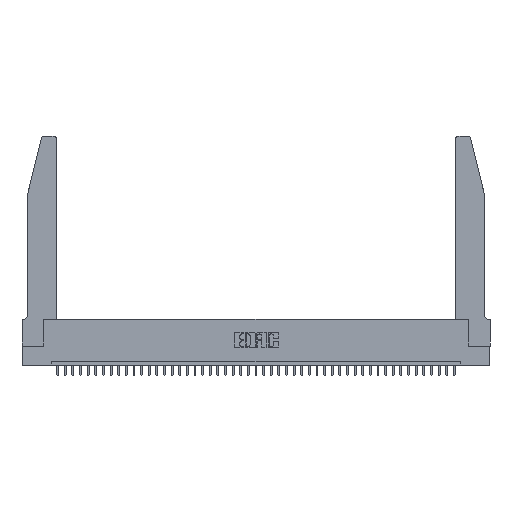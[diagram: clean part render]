
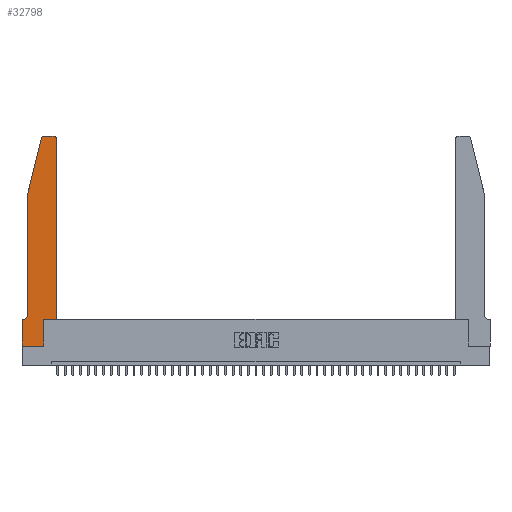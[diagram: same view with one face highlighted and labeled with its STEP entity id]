
A CAD part, top view. The second image highlights one B-rep face of the part: STEP entity #32798.
In plain terms, the highlighted planar face has unit normal (0, 0, 1).
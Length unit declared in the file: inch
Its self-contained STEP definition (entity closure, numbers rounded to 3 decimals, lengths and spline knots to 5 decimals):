
#732 = CARTESIAN_POINT ( 'NONE',  ( 0.0755, 2., 0.37 ) ) ;
#1576 = CARTESIAN_POINT ( 'NONE',  ( 0.4505, 0.35, 0.37 ) ) ;
#1791 = CARTESIAN_POINT ( 'NONE',  ( 0., 0., 0.37 ) ) ;
#2016 = ORIENTED_EDGE ( 'NONE', *, *, #5749, .T. ) ;
#2345 = CARTESIAN_POINT ( 'NONE',  ( 0.0055, 0.42, 0.37 ) ) ;
#2664 = ORIENTED_EDGE ( 'NONE', *, *, #18466, .T. ) ;
#3115 = EDGE_CURVE ( 'NONE', #24210, #10207, #22280, .T. ) ;
#3651 = AXIS2_PLACEMENT_3D ( 'NONE', #23842, #14091, #20519 ) ;
#4478 = CARTESIAN_POINT ( 'NONE',  ( 0.2865, 0.35, 0.37 ) ) ;
#4859 = VECTOR ( 'NONE', #13018, 39.37008 ) ;
#5281 = LINE ( 'NONE', #4478, #11576 ) ;
#5500 = DIRECTION ( 'NONE',  ( 0., -1., 0. ) ) ;
#5743 = ORIENTED_EDGE ( 'NONE', *, *, #36194, .T. ) ;
#5749 = EDGE_CURVE ( 'NONE', #22017, #24210, #34456, .T. ) ;
#5859 = DIRECTION ( 'NONE',  ( 0., 0., 1. ) ) ;
#6231 = VECTOR ( 'NONE', #37303, 39.37008 ) ;
#6302 = CARTESIAN_POINT ( 'NONE',  ( 0.4205, 2.75, 0.37 ) ) ;
#6963 = ORIENTED_EDGE ( 'NONE', *, *, #41807, .T. ) ;
#7264 = CIRCLE ( 'NONE', #24966, 0.07 ) ;
#8176 = DIRECTION ( 'NONE',  ( -1., 0., 0. ) ) ;
#8345 = CARTESIAN_POINT ( 'NONE',  ( 0.0055, 0.35, 0.37 ) ) ;
#8412 = CARTESIAN_POINT ( 'NONE',  ( 0.2865, 0., 0.37 ) ) ;
#8588 = ORIENTED_EDGE ( 'NONE', *, *, #36575, .T. ) ;
#9119 = VECTOR ( 'NONE', #8176, 39.37008 ) ;
#10207 = VERTEX_POINT ( 'NONE', #8412 ) ;
#10593 = VERTEX_POINT ( 'NONE', #8345 ) ;
#10775 = CARTESIAN_POINT ( 'NONE',  ( 0., 0., 0.37 ) ) ;
#10812 = AXIS2_PLACEMENT_3D ( 'NONE', #13047, #5859, #29155 ) ;
#11576 = VECTOR ( 'NONE', #31412, 39.37008 ) ;
#12307 = DIRECTION ( 'NONE',  ( 0., 0., 1. ) ) ;
#12353 = ORIENTED_EDGE ( 'NONE', *, *, #13161, .T. ) ;
#13018 = DIRECTION ( 'NONE',  ( 0., 1., 0. ) ) ;
#13047 = CARTESIAN_POINT ( 'NONE',  ( 0., 0.35, 0.37 ) ) ;
#13161 = EDGE_CURVE ( 'NONE', #34964, #14370, #29310, .T. ) ;
#13589 = ORIENTED_EDGE ( 'NONE', *, *, #20872, .T. ) ;
#13642 = DIRECTION ( 'NONE',  ( -0.239, -0.971, 0. ) ) ;
#14087 = LINE ( 'NONE', #37726, #6231 ) ;
#14091 = DIRECTION ( 'NONE',  ( 0., 0., 1. ) ) ;
#14370 = VERTEX_POINT ( 'NONE', #6302 ) ;
#15815 = ORIENTED_EDGE ( 'NONE', *, *, #22058, .T. ) ;
#16415 = DIRECTION ( 'NONE',  ( 0., 0., -1. ) ) ;
#16569 = DIRECTION ( 'NONE',  ( 1., 0., 0. ) ) ;
#16833 = VECTOR ( 'NONE', #18344, 39.37008 ) ;
#16933 = VECTOR ( 'NONE', #5500, 39.37008 ) ;
#18344 = DIRECTION ( 'NONE',  ( 0., -1., 0. ) ) ;
#18466 = EDGE_CURVE ( 'NONE', #10593, #22017, #35674, .T. ) ;
#18533 = CARTESIAN_POINT ( 'NONE',  ( 0.0755, 2., 0.37 ) ) ;
#18582 = LINE ( 'NONE', #35150, #35183 ) ;
#18977 = VERTEX_POINT ( 'NONE', #26838 ) ;
#19593 = VECTOR ( 'NONE', #13642, 39.37008 ) ;
#20417 = DIRECTION ( 'NONE',  ( 1., 0., 0. ) ) ;
#20519 = DIRECTION ( 'NONE',  ( 1., 0., 0. ) ) ;
#20576 = LINE ( 'NONE', #28409, #4859 ) ;
#20754 = VECTOR ( 'NONE', #20417, 39.37008 ) ;
#20872 = EDGE_CURVE ( 'NONE', #10207, #18977, #5281, .T. ) ;
#22017 = VERTEX_POINT ( 'NONE', #33407 ) ;
#22058 = EDGE_CURVE ( 'NONE', #14370, #34557, #14087, .T. ) ;
#22280 = LINE ( 'NONE', #10775, #20754 ) ;
#22322 = CARTESIAN_POINT ( 'NONE',  ( 0.0755, 2., 0.37 ) ) ;
#22649 = CARTESIAN_POINT ( 'NONE',  ( 0.4205, 2.72, 0.37 ) ) ;
#23131 = ORIENTED_EDGE ( 'NONE', *, *, #28394, .T. ) ;
#23842 = CARTESIAN_POINT ( 'NONE',  ( 0.284, 2.72, 0.37 ) ) ;
#24210 = VERTEX_POINT ( 'NONE', #38657 ) ;
#24966 = AXIS2_PLACEMENT_3D ( 'NONE', #2345, #16415, #42419 ) ;
#25112 = ORIENTED_EDGE ( 'NONE', *, *, #30130, .T. ) ;
#25743 = LINE ( 'NONE', #18533, #16933 ) ;
#26838 = CARTESIAN_POINT ( 'NONE',  ( 0.2865, 0.35, 0.37 ) ) ;
#27504 = VERTEX_POINT ( 'NONE', #22322 ) ;
#27715 = CARTESIAN_POINT ( 'NONE',  ( 0.0755, 0.42, 0.37 ) ) ;
#27795 = CARTESIAN_POINT ( 'NONE',  ( 0.25487, 2.72718, 0.37 ) ) ;
#28394 = EDGE_CURVE ( 'NONE', #34557, #40960, #31785, .T. ) ;
#28409 = CARTESIAN_POINT ( 'NONE',  ( 0.4505, 0.35, 0.37 ) ) ;
#29155 = DIRECTION ( 'NONE',  ( 1., 0., 0. ) ) ;
#29310 = CIRCLE ( 'NONE', #30881, 0.03 ) ;
#30130 = EDGE_CURVE ( 'NONE', #42109, #10593, #7264, .T. ) ;
#30881 = AXIS2_PLACEMENT_3D ( 'NONE', #22649, #12307, #16569 ) ;
#31007 = FACE_OUTER_BOUND ( 'NONE', #38969, .T. ) ;
#31412 = DIRECTION ( 'NONE',  ( 0., 1., 0. ) ) ;
#31785 = CIRCLE ( 'NONE', #3651, 0.03 ) ;
#32798 = ADVANCED_FACE ( 'NONE', ( #31007 ), #32942, .T. ) ;
#32942 = PLANE ( 'NONE',  #10812 ) ;
#33059 = LINE ( 'NONE', #732, #19593 ) ;
#33407 = CARTESIAN_POINT ( 'NONE',  ( 0., 0.35, 0.37 ) ) ;
#34151 = ORIENTED_EDGE ( 'NONE', *, *, #3115, .T. ) ;
#34456 = LINE ( 'NONE', #1791, #16833 ) ;
#34557 = VERTEX_POINT ( 'NONE', #35099 ) ;
#34964 = VERTEX_POINT ( 'NONE', #41437 ) ;
#35099 = CARTESIAN_POINT ( 'NONE',  ( 0.284, 2.75, 0.37 ) ) ;
#35150 = CARTESIAN_POINT ( 'NONE',  ( 0.4505, 0.35, 0.37 ) ) ;
#35183 = VECTOR ( 'NONE', #38358, 39.37008 ) ;
#35674 = LINE ( 'NONE', #41388, #9119 ) ;
#36194 = EDGE_CURVE ( 'NONE', #40960, #27504, #33059, .T. ) ;
#36575 = EDGE_CURVE ( 'NONE', #39130, #34964, #20576, .T. ) ;
#36947 = EDGE_CURVE ( 'NONE', #27504, #42109, #25743, .T. ) ;
#37303 = DIRECTION ( 'NONE',  ( -1., 0., 0. ) ) ;
#37726 = CARTESIAN_POINT ( 'NONE',  ( 0.2605, 2.75, 0.37 ) ) ;
#38358 = DIRECTION ( 'NONE',  ( 1., 0., 0. ) ) ;
#38657 = CARTESIAN_POINT ( 'NONE',  ( 0., 0., 0.37 ) ) ;
#38969 = EDGE_LOOP ( 'NONE', ( #15815, #23131, #5743, #40442, #25112, #2664, #2016, #34151, #13589, #6963, #8588, #12353 ) ) ;
#39130 = VERTEX_POINT ( 'NONE', #1576 ) ;
#40442 = ORIENTED_EDGE ( 'NONE', *, *, #36947, .T. ) ;
#40960 = VERTEX_POINT ( 'NONE', #27795 ) ;
#41388 = CARTESIAN_POINT ( 'NONE',  ( 0.0755, 0.35, 0.37 ) ) ;
#41437 = CARTESIAN_POINT ( 'NONE',  ( 0.4505, 2.72, 0.37 ) ) ;
#41807 = EDGE_CURVE ( 'NONE', #18977, #39130, #18582, .T. ) ;
#42109 = VERTEX_POINT ( 'NONE', #27715 ) ;
#42419 = DIRECTION ( 'NONE',  ( -1., 0., 0. ) ) ;
